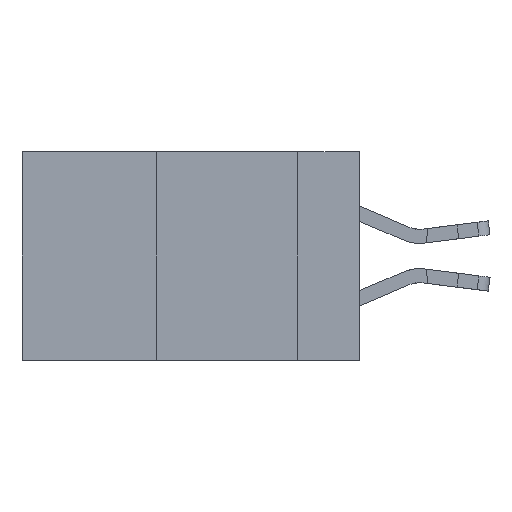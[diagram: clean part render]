
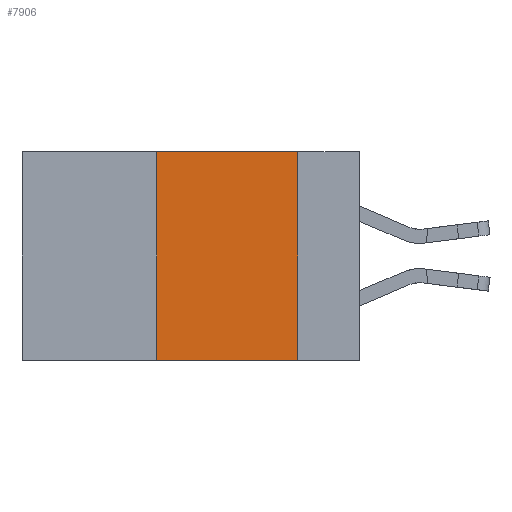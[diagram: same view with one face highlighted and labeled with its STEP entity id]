
A CAD part, left-side view. The second image highlights one B-rep face of the part: STEP entity #7906.
In plain terms, the highlighted planar face has unit normal (-1, 0, 0).
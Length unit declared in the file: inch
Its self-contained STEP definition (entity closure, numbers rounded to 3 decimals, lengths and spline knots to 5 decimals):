
#87 = VERTEX_POINT ( 'NONE', #5551 ) ;
#543 = LINE ( 'NONE', #6088, #12011 ) ;
#776 = DIRECTION ( 'NONE',  ( 1., 0., 0. ) ) ;
#990 = CARTESIAN_POINT ( 'NONE',  ( 0., 0.6, -0.37 ) ) ;
#1098 = CARTESIAN_POINT ( 'NONE',  ( 0., 0.36, 0. ) ) ;
#1519 = DIRECTION ( 'NONE',  ( 0., -1., 0. ) ) ;
#2229 = EDGE_CURVE ( 'NONE', #12998, #2281, #17172, .T. ) ;
#2281 = VERTEX_POINT ( 'NONE', #14997 ) ;
#2608 = DIRECTION ( 'NONE',  ( 0., -1., 0. ) ) ;
#3596 = CARTESIAN_POINT ( 'NONE',  ( 0., 0.36, -0.37 ) ) ;
#3884 = VERTEX_POINT ( 'NONE', #14026 ) ;
#5551 = CARTESIAN_POINT ( 'NONE',  ( 0., 0.11, 0. ) ) ;
#5742 = EDGE_CURVE ( 'NONE', #87, #3884, #543, .T. ) ;
#6088 = CARTESIAN_POINT ( 'NONE',  ( 0., 0.11, 0. ) ) ;
#6238 = VECTOR ( 'NONE', #1519, 39.37008 ) ;
#6715 = ORIENTED_EDGE ( 'NONE', *, *, #5742, .F. ) ;
#7906 = ADVANCED_FACE ( 'NONE', ( #11989 ), #10171, .F. ) ;
#7957 = AXIS2_PLACEMENT_3D ( 'NONE', #8582, #776, #11686 ) ;
#8582 = CARTESIAN_POINT ( 'NONE',  ( 0., 0.6, 0. ) ) ;
#8956 = VECTOR ( 'NONE', #2608, 39.37008 ) ;
#9301 = CARTESIAN_POINT ( 'NONE',  ( 0., 0.6, 0. ) ) ;
#9345 = DIRECTION ( 'NONE',  ( 0., 0., -1. ) ) ;
#10154 = ORIENTED_EDGE ( 'NONE', *, *, #11359, .T. ) ;
#10171 = PLANE ( 'NONE',  #7957 ) ;
#11359 = EDGE_CURVE ( 'NONE', #12998, #3884, #13443, .T. ) ;
#11686 = DIRECTION ( 'NONE',  ( 0., 0., -1. ) ) ;
#11989 = FACE_OUTER_BOUND ( 'NONE', #18534, .T. ) ;
#12011 = VECTOR ( 'NONE', #9345, 39.37008 ) ;
#12998 = VERTEX_POINT ( 'NONE', #3596 ) ;
#13270 = VECTOR ( 'NONE', #19278, 39.37008 ) ;
#13443 = LINE ( 'NONE', #990, #8956 ) ;
#14026 = CARTESIAN_POINT ( 'NONE',  ( 0., 0.11, -0.37 ) ) ;
#14997 = CARTESIAN_POINT ( 'NONE',  ( 0., 0.36, 0. ) ) ;
#15254 = ORIENTED_EDGE ( 'NONE', *, *, #19209, .F. ) ;
#17080 = ORIENTED_EDGE ( 'NONE', *, *, #2229, .F. ) ;
#17172 = LINE ( 'NONE', #1098, #13270 ) ;
#18245 = LINE ( 'NONE', #9301, #6238 ) ;
#18534 = EDGE_LOOP ( 'NONE', ( #6715, #15254, #17080, #10154 ) ) ;
#19209 = EDGE_CURVE ( 'NONE', #2281, #87, #18245, .T. ) ;
#19278 = DIRECTION ( 'NONE',  ( 0., 0., 1. ) ) ;
